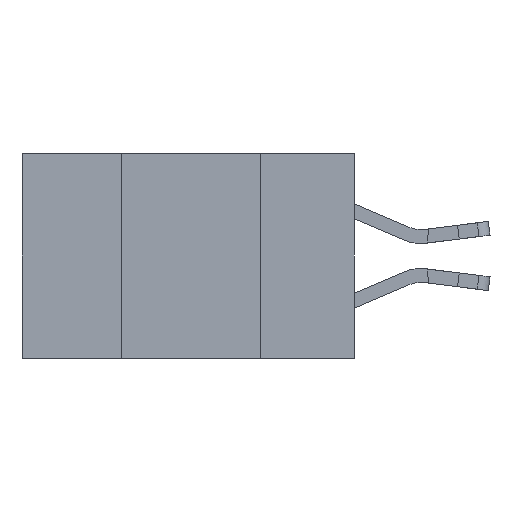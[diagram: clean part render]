
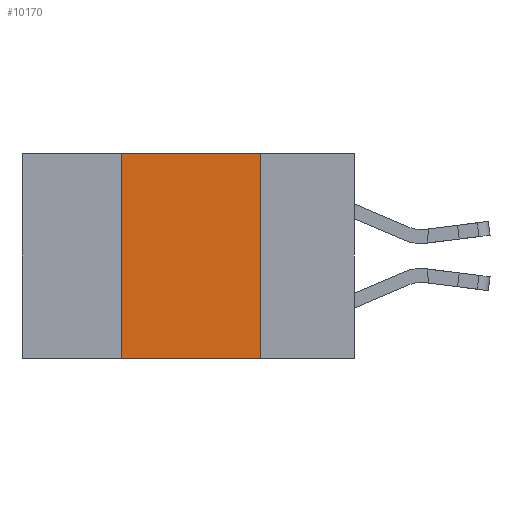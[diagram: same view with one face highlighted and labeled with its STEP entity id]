
A CAD part, left-side view. The second image highlights one B-rep face of the part: STEP entity #10170.
In plain terms, the highlighted planar face has unit normal (-1, 0, 0).
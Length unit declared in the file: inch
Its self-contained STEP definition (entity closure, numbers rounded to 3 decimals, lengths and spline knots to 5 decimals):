
#46 = PLANE ( 'NONE',  #3245 ) ;
#612 = CARTESIAN_POINT ( 'NONE',  ( 0., 0.17, 0. ) ) ;
#1026 = EDGE_CURVE ( 'NONE', #5696, #2776, #10859, .T. ) ;
#1530 = DIRECTION ( 'NONE',  ( 0., -1., 0. ) ) ;
#1805 = VERTEX_POINT ( 'NONE', #8012 ) ;
#2273 = ORIENTED_EDGE ( 'NONE', *, *, #1026, .F. ) ;
#2776 = VERTEX_POINT ( 'NONE', #10688 ) ;
#2792 = DIRECTION ( 'NONE',  ( 0., 0., 1. ) ) ;
#3245 = AXIS2_PLACEMENT_3D ( 'NONE', #11477, #5833, #10435 ) ;
#3533 = VECTOR ( 'NONE', #7553, 39.37008 ) ;
#4530 = FACE_OUTER_BOUND ( 'NONE', #12438, .T. ) ;
#4793 = CARTESIAN_POINT ( 'NONE',  ( 0., 0.6, 0. ) ) ;
#5695 = ORIENTED_EDGE ( 'NONE', *, *, #9502, .F. ) ;
#5696 = VERTEX_POINT ( 'NONE', #13807 ) ;
#5833 = DIRECTION ( 'NONE',  ( 1., 0., 0. ) ) ;
#5848 = DIRECTION ( 'NONE',  ( 0., -1., 0. ) ) ;
#6589 = VECTOR ( 'NONE', #5848, 39.37008 ) ;
#7553 = DIRECTION ( 'NONE',  ( 0., 0., -1. ) ) ;
#7653 = LINE ( 'NONE', #612, #3533 ) ;
#8012 = CARTESIAN_POINT ( 'NONE',  ( 0., 0.42, -0.37 ) ) ;
#8503 = CARTESIAN_POINT ( 'NONE',  ( 0., 0.42, 0. ) ) ;
#8911 = CARTESIAN_POINT ( 'NONE',  ( 0., 0.17, -0.37 ) ) ;
#9502 = EDGE_CURVE ( 'NONE', #2776, #11056, #7653, .T. ) ;
#10170 = ADVANCED_FACE ( 'NONE', ( #4530 ), #46, .F. ) ;
#10222 = VECTOR ( 'NONE', #2792, 39.37008 ) ;
#10386 = LINE ( 'NONE', #10645, #13615 ) ;
#10435 = DIRECTION ( 'NONE',  ( 0., 0., -1. ) ) ;
#10645 = CARTESIAN_POINT ( 'NONE',  ( 0., 0.6, -0.37 ) ) ;
#10688 = CARTESIAN_POINT ( 'NONE',  ( 0., 0.17, 0. ) ) ;
#10859 = LINE ( 'NONE', #4793, #6589 ) ;
#11056 = VERTEX_POINT ( 'NONE', #8911 ) ;
#11187 = EDGE_CURVE ( 'NONE', #1805, #5696, #12180, .T. ) ;
#11477 = CARTESIAN_POINT ( 'NONE',  ( 0., 0.6, 0. ) ) ;
#11533 = EDGE_CURVE ( 'NONE', #1805, #11056, #10386, .T. ) ;
#12180 = LINE ( 'NONE', #8503, #10222 ) ;
#12438 = EDGE_LOOP ( 'NONE', ( #5695, #2273, #14622, #12570 ) ) ;
#12570 = ORIENTED_EDGE ( 'NONE', *, *, #11533, .T. ) ;
#13615 = VECTOR ( 'NONE', #1530, 39.37008 ) ;
#13807 = CARTESIAN_POINT ( 'NONE',  ( 0., 0.42, 0. ) ) ;
#14622 = ORIENTED_EDGE ( 'NONE', *, *, #11187, .F. ) ;
